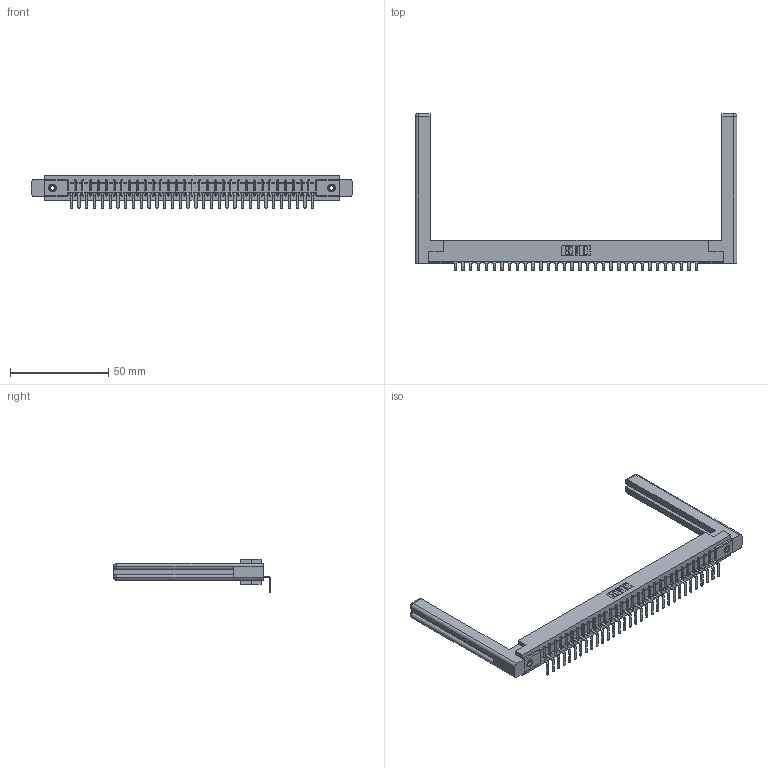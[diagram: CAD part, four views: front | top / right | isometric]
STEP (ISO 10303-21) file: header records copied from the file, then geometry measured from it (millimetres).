
FILE_DESCRIPTION (( 'STEP AP203' ), '1' );
FILE_NAME ('307-032-559-158.STEP', '2019-09-05T16:38:24', ( '' ), ( '' ), 'SwSTEP 2.0', 'SolidWorks 2016', '' );
FILE_SCHEMA (( 'CONFIG_CONTROL_DESIGN' ));
Length unit declared in the file: inch
Products named in the file (5): 307-032-559-158; 345-250-001_345-250-001-102; 307-290-001_558 559 - 1 (Single); 307 Part_.156 Dia Mounting Holes; 307-220-058
Assembly tree (37 placements, depth 2):
  307-032-559-158
    307 Part_.156 Dia Mounting Holes
    307-290-001_558 559 - 1 (Single)  x32
    307-220-058  x2
    345-250-001_345-250-001-102  x2
Bounding box: 163.42 x 79.77 x 16.8 mm (x, y, z)
Volume: 24111.3 mm3; surface area: 23228.8 mm2
Topology: 37 solids, 37 shells, 2213 faces, 6245 edges, 4018 vertices
Faces by surface type: plane 1402, cylinder 721, sphere 66, torus 12, cone 12
Entity records: 31403 total; most frequent: CARTESIAN_POINT 5295, ORIENTED_EDGE 5220, DIRECTION 5116, EDGE_CURVE 2610, VECTOR 1994, LINE 1994, VERTEX_POINT 1686, AXIS2_PLACEMENT_3D 1561
